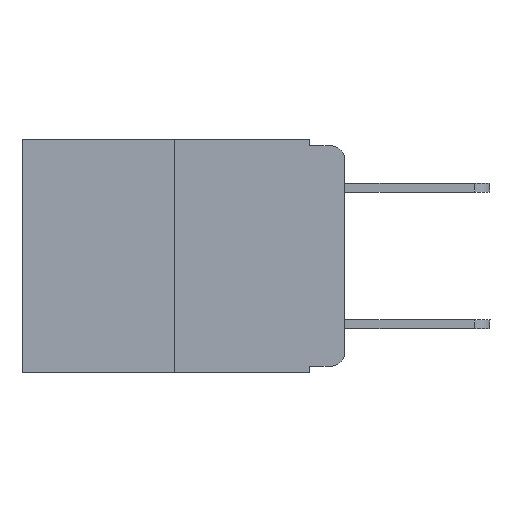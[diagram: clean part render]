
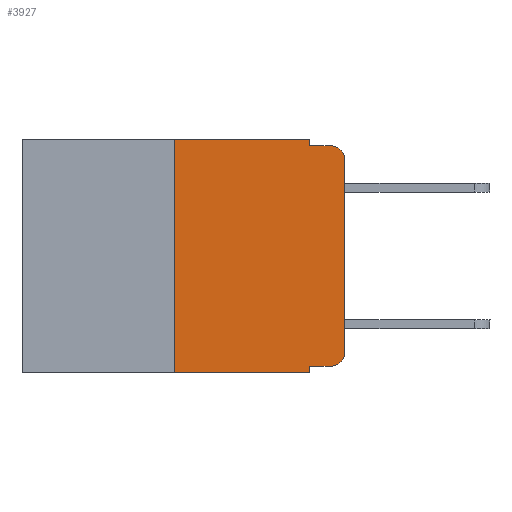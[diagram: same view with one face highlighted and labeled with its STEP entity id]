
A CAD part, left-side view. The second image highlights one B-rep face of the part: STEP entity #3927.
In plain terms, the highlighted planar face has unit normal (-1, 0, 0).
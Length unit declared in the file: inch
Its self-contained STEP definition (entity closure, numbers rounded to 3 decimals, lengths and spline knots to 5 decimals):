
#15 = VERTEX_POINT ( 'NONE', #3580 ) ;
#18 = CARTESIAN_POINT ( 'NONE',  ( 0., 0., 0. ) ) ;
#430 = AXIS2_PLACEMENT_3D ( 'NONE', #1896, #13006, #1764 ) ;
#606 = AXIS2_PLACEMENT_3D ( 'NONE', #12650, #6547, #9759 ) ;
#649 = ORIENTED_EDGE ( 'NONE', *, *, #8810, .F. ) ;
#928 = DIRECTION ( 'NONE',  ( 0., -1., 0. ) ) ;
#999 = ORIENTED_EDGE ( 'NONE', *, *, #12908, .T. ) ;
#1134 = ORIENTED_EDGE ( 'NONE', *, *, #6503, .T. ) ;
#1239 = CIRCLE ( 'NONE', #606, 0.02 ) ;
#1458 = DIRECTION ( 'NONE',  ( 0., 0., -1. ) ) ;
#1657 = DIRECTION ( 'NONE',  ( 0., 0., 1. ) ) ;
#1764 = DIRECTION ( 'NONE',  ( 0., 0., -1. ) ) ;
#1768 = EDGE_CURVE ( 'NONE', #3942, #15, #10535, .T. ) ;
#1896 = CARTESIAN_POINT ( 'NONE',  ( 0., 0.473, 0. ) ) ;
#2038 = VERTEX_POINT ( 'NONE', #12459 ) ;
#2049 = VERTEX_POINT ( 'NONE', #6028 ) ;
#2226 = VERTEX_POINT ( 'NONE', #9558 ) ;
#2438 = ORIENTED_EDGE ( 'NONE', *, *, #4340, .T. ) ;
#2586 = DIRECTION ( 'NONE',  ( 0., -1., 0. ) ) ;
#2611 = VERTEX_POINT ( 'NONE', #11486 ) ;
#2614 = ORIENTED_EDGE ( 'NONE', *, *, #11893, .F. ) ;
#2632 = ORIENTED_EDGE ( 'NONE', *, *, #6782, .T. ) ;
#2721 = LINE ( 'NONE', #2789, #12732 ) ;
#2789 = CARTESIAN_POINT ( 'NONE',  ( 0., 0.25, 0. ) ) ;
#3580 = CARTESIAN_POINT ( 'NONE',  ( 0., 0.051, -0.343 ) ) ;
#3654 = LINE ( 'NONE', #11544, #7563 ) ;
#3854 = VECTOR ( 'NONE', #928, 39.37008 ) ;
#3927 = ADVANCED_FACE ( 'NONE', ( #7821 ), #11048, .F. ) ;
#3942 = VERTEX_POINT ( 'NONE', #9154 ) ;
#3973 = VERTEX_POINT ( 'NONE', #6018 ) ;
#4028 = CARTESIAN_POINT ( 'NONE',  ( 0., 0.02, -0.313 ) ) ;
#4038 = DIRECTION ( 'NONE',  ( 0., 0., 1. ) ) ;
#4340 = EDGE_CURVE ( 'NONE', #2226, #15, #4996, .T. ) ;
#4371 = CARTESIAN_POINT ( 'NONE',  ( 0., 0.051, -0.01 ) ) ;
#4463 = CARTESIAN_POINT ( 'NONE',  ( 0., 0.051, 0. ) ) ;
#4996 = LINE ( 'NONE', #9052, #9174 ) ;
#5634 = ORIENTED_EDGE ( 'NONE', *, *, #1768, .F. ) ;
#5928 = CIRCLE ( 'NONE', #9117, 0.02 ) ;
#6018 = CARTESIAN_POINT ( 'NONE',  ( 0., 0.051, 0. ) ) ;
#6028 = CARTESIAN_POINT ( 'NONE',  ( 0., 0.02, -0.333 ) ) ;
#6497 = VERTEX_POINT ( 'NONE', #13069 ) ;
#6503 = EDGE_CURVE ( 'NONE', #2049, #2611, #5928, .T. ) ;
#6547 = DIRECTION ( 'NONE',  ( -1., 0., 0. ) ) ;
#6782 = EDGE_CURVE ( 'NONE', #11624, #6497, #1239, .T. ) ;
#6886 = DIRECTION ( 'NONE',  ( 0., -1., 0. ) ) ;
#7563 = VECTOR ( 'NONE', #2586, 39.37008 ) ;
#7701 = ORIENTED_EDGE ( 'NONE', *, *, #13169, .F. ) ;
#7821 = FACE_OUTER_BOUND ( 'NONE', #10864, .T. ) ;
#8512 = CARTESIAN_POINT ( 'NONE',  ( 0., 0.051, 0. ) ) ;
#8810 = EDGE_CURVE ( 'NONE', #10759, #6497, #8935, .T. ) ;
#8935 = LINE ( 'NONE', #8997, #3854 ) ;
#8997 = CARTESIAN_POINT ( 'NONE',  ( 0., 0.051, -0.01 ) ) ;
#9025 = DIRECTION ( 'NONE',  ( -1., 0., 0. ) ) ;
#9052 = CARTESIAN_POINT ( 'NONE',  ( 0., 0.473, -0.343 ) ) ;
#9117 = AXIS2_PLACEMENT_3D ( 'NONE', #4028, #9025, #10178 ) ;
#9154 = CARTESIAN_POINT ( 'NONE',  ( 0., 0.051, -0.333 ) ) ;
#9174 = VECTOR ( 'NONE', #13159, 39.37008 ) ;
#9321 = DIRECTION ( 'NONE',  ( 0., 0., -1. ) ) ;
#9558 = CARTESIAN_POINT ( 'NONE',  ( 0., 0.25, -0.343 ) ) ;
#9665 = CARTESIAN_POINT ( 'NONE',  ( 0., 0., -0.03 ) ) ;
#9691 = ORIENTED_EDGE ( 'NONE', *, *, #12097, .F. ) ;
#9699 = LINE ( 'NONE', #12926, #10822 ) ;
#9759 = DIRECTION ( 'NONE',  ( 0., 0., -1. ) ) ;
#10178 = DIRECTION ( 'NONE',  ( 0., 0., -1. ) ) ;
#10238 = ORIENTED_EDGE ( 'NONE', *, *, #12672, .T. ) ;
#10377 = VECTOR ( 'NONE', #4038, 39.37008 ) ;
#10535 = LINE ( 'NONE', #8512, #12457 ) ;
#10759 = VERTEX_POINT ( 'NONE', #4371 ) ;
#10822 = VECTOR ( 'NONE', #6886, 39.37008 ) ;
#10864 = EDGE_LOOP ( 'NONE', ( #10238, #2632, #649, #7701, #2614, #9691, #2438, #5634, #999, #1134 ) ) ;
#11048 = PLANE ( 'NONE',  #430 ) ;
#11486 = CARTESIAN_POINT ( 'NONE',  ( 0., 0., -0.313 ) ) ;
#11544 = CARTESIAN_POINT ( 'NONE',  ( 0., 0.473, 0. ) ) ;
#11546 = LINE ( 'NONE', #4463, #12533 ) ;
#11624 = VERTEX_POINT ( 'NONE', #9665 ) ;
#11893 = EDGE_CURVE ( 'NONE', #2038, #3973, #3654, .T. ) ;
#12097 = EDGE_CURVE ( 'NONE', #2226, #2038, #2721, .T. ) ;
#12457 = VECTOR ( 'NONE', #9321, 39.37008 ) ;
#12459 = CARTESIAN_POINT ( 'NONE',  ( 0., 0.25, 0. ) ) ;
#12533 = VECTOR ( 'NONE', #1458, 39.37008 ) ;
#12650 = CARTESIAN_POINT ( 'NONE',  ( 0., 0.02, -0.03 ) ) ;
#12672 = EDGE_CURVE ( 'NONE', #2611, #11624, #13210, .T. ) ;
#12732 = VECTOR ( 'NONE', #1657, 39.37008 ) ;
#12908 = EDGE_CURVE ( 'NONE', #3942, #2049, #9699, .T. ) ;
#12926 = CARTESIAN_POINT ( 'NONE',  ( 0., 0.051, -0.333 ) ) ;
#13006 = DIRECTION ( 'NONE',  ( 1., 0., 0. ) ) ;
#13069 = CARTESIAN_POINT ( 'NONE',  ( 0., 0.02, -0.01 ) ) ;
#13159 = DIRECTION ( 'NONE',  ( 0., -1., 0. ) ) ;
#13169 = EDGE_CURVE ( 'NONE', #3973, #10759, #11546, .T. ) ;
#13210 = LINE ( 'NONE', #18, #10377 ) ;
